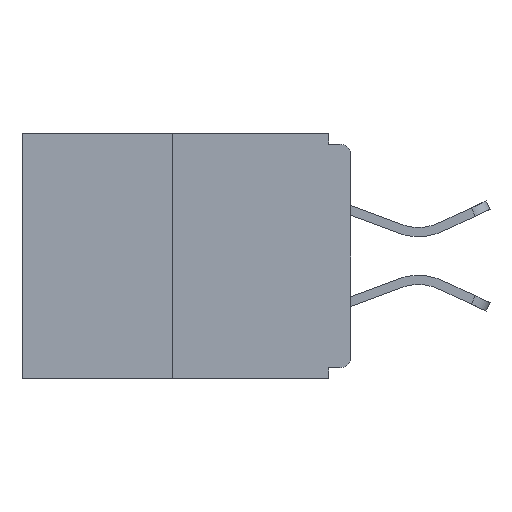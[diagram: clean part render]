
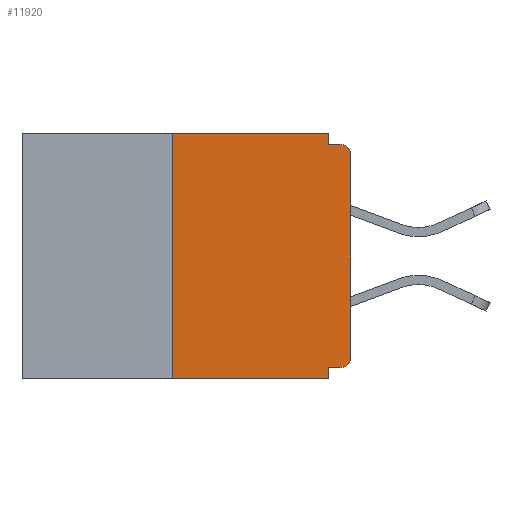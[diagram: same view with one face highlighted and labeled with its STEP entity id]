
A CAD part, left-side view. The second image highlights one B-rep face of the part: STEP entity #11920.
In plain terms, the highlighted planar face has unit normal (-1, 0, 0).
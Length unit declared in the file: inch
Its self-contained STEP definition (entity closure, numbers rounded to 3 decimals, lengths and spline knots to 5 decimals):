
#701 = CIRCLE ( 'NONE', #27333, 0.015 ) ;
#1292 = VERTEX_POINT ( 'NONE', #9075 ) ;
#2211 = CARTESIAN_POINT ( 'NONE',  ( 0., 0.25, 0. ) ) ;
#2224 = CARTESIAN_POINT ( 'NONE',  ( 0., 0.031, -0.015 ) ) ;
#3467 = VERTEX_POINT ( 'NONE', #19115 ) ;
#3936 = EDGE_CURVE ( 'NONE', #1292, #20335, #16505, .T. ) ;
#4167 = EDGE_CURVE ( 'NONE', #28776, #17093, #6380, .T. ) ;
#4776 = CARTESIAN_POINT ( 'NONE',  ( 0., 0.031, 0. ) ) ;
#5750 = CIRCLE ( 'NONE', #9636, 0.015 ) ;
#6220 = DIRECTION ( 'NONE',  ( 0., 0., 1. ) ) ;
#6380 = LINE ( 'NONE', #16462, #31080 ) ;
#6682 = CARTESIAN_POINT ( 'NONE',  ( 0., 0.031, 0. ) ) ;
#6690 = EDGE_CURVE ( 'NONE', #9240, #1292, #701, .T. ) ;
#6781 = VECTOR ( 'NONE', #25432, 39.37008 ) ;
#7291 = ORIENTED_EDGE ( 'NONE', *, *, #4167, .T. ) ;
#7718 = EDGE_CURVE ( 'NONE', #3467, #17093, #22141, .T. ) ;
#8162 = VECTOR ( 'NONE', #19704, 39.37008 ) ;
#8399 = LINE ( 'NONE', #25861, #15751 ) ;
#9075 = CARTESIAN_POINT ( 'NONE',  ( 0., 0., -0.313 ) ) ;
#9240 = VERTEX_POINT ( 'NONE', #25787 ) ;
#9314 = EDGE_CURVE ( 'NONE', #31200, #23020, #10562, .T. ) ;
#9426 = CARTESIAN_POINT ( 'NONE',  ( 0., 0.015, -0.313 ) ) ;
#9548 = CARTESIAN_POINT ( 'NONE',  ( 0., 0.031, -0.343 ) ) ;
#9636 = AXIS2_PLACEMENT_3D ( 'NONE', #28320, #13290, #18084 ) ;
#10562 = LINE ( 'NONE', #6682, #29783 ) ;
#11920 = ADVANCED_FACE ( 'NONE', ( #14346 ), #28567, .F. ) ;
#12516 = ORIENTED_EDGE ( 'NONE', *, *, #15513, .F. ) ;
#13290 = DIRECTION ( 'NONE',  ( -1., 0., 0. ) ) ;
#13300 = CARTESIAN_POINT ( 'NONE',  ( 0., 0.46, 0. ) ) ;
#13305 = VERTEX_POINT ( 'NONE', #31571 ) ;
#13986 = DIRECTION ( 'NONE',  ( 1., 0., 0. ) ) ;
#14346 = FACE_OUTER_BOUND ( 'NONE', #15248, .T. ) ;
#14464 = AXIS2_PLACEMENT_3D ( 'NONE', #26208, #13986, #16027 ) ;
#15248 = EDGE_LOOP ( 'NONE', ( #20607, #30064, #7291, #23464, #16384, #20181, #25159, #20839, #12516, #31578 ) ) ;
#15513 = EDGE_CURVE ( 'NONE', #23020, #13305, #8399, .T. ) ;
#15751 = VECTOR ( 'NONE', #30982, 39.37008 ) ;
#15843 = VERTEX_POINT ( 'NONE', #2211 ) ;
#16027 = DIRECTION ( 'NONE',  ( 0., 0., -1. ) ) ;
#16252 = EDGE_CURVE ( 'NONE', #15843, #31200, #31839, .T. ) ;
#16319 = DIRECTION ( 'NONE',  ( 0., 0., -1. ) ) ;
#16384 = ORIENTED_EDGE ( 'NONE', *, *, #29348, .F. ) ;
#16462 = CARTESIAN_POINT ( 'NONE',  ( 0., 0.46, -0.343 ) ) ;
#16505 = LINE ( 'NONE', #31599, #29852 ) ;
#17093 = VERTEX_POINT ( 'NONE', #9548 ) ;
#17262 = CARTESIAN_POINT ( 'NONE',  ( 0., 0.25, 0. ) ) ;
#18084 = DIRECTION ( 'NONE',  ( 0., 0., -1. ) ) ;
#18687 = DIRECTION ( 'NONE',  ( 0., 0., -1. ) ) ;
#18782 = DIRECTION ( 'NONE',  ( 0., 1., 0. ) ) ;
#19115 = CARTESIAN_POINT ( 'NONE',  ( 0., 0.031, -0.328 ) ) ;
#19704 = DIRECTION ( 'NONE',  ( 0., 0., 1. ) ) ;
#20181 = ORIENTED_EDGE ( 'NONE', *, *, #6690, .T. ) ;
#20218 = EDGE_CURVE ( 'NONE', #20335, #13305, #5750, .T. ) ;
#20232 = LINE ( 'NONE', #17262, #8162 ) ;
#20335 = VERTEX_POINT ( 'NONE', #24767 ) ;
#20580 = VECTOR ( 'NONE', #16319, 39.37008 ) ;
#20607 = ORIENTED_EDGE ( 'NONE', *, *, #16252, .F. ) ;
#20839 = ORIENTED_EDGE ( 'NONE', *, *, #20218, .T. ) ;
#21516 = DIRECTION ( 'NONE',  ( 0., -1., 0. ) ) ;
#22141 = LINE ( 'NONE', #30966, #20580 ) ;
#23020 = VERTEX_POINT ( 'NONE', #2224 ) ;
#23464 = ORIENTED_EDGE ( 'NONE', *, *, #7718, .F. ) ;
#23481 = CARTESIAN_POINT ( 'NONE',  ( 0., 0., -0.328 ) ) ;
#24767 = CARTESIAN_POINT ( 'NONE',  ( 0., 0., -0.03 ) ) ;
#25159 = ORIENTED_EDGE ( 'NONE', *, *, #3936, .T. ) ;
#25432 = DIRECTION ( 'NONE',  ( 0., -1., 0. ) ) ;
#25787 = CARTESIAN_POINT ( 'NONE',  ( 0., 0.015, -0.328 ) ) ;
#25789 = VECTOR ( 'NONE', #18782, 39.37008 ) ;
#25861 = CARTESIAN_POINT ( 'NONE',  ( 0., 0., -0.015 ) ) ;
#26208 = CARTESIAN_POINT ( 'NONE',  ( 0., 0.46, 0. ) ) ;
#27029 = CARTESIAN_POINT ( 'NONE',  ( 0., 0.25, -0.343 ) ) ;
#27333 = AXIS2_PLACEMENT_3D ( 'NONE', #9426, #27467, #31881 ) ;
#27467 = DIRECTION ( 'NONE',  ( -1., 0., 0. ) ) ;
#28320 = CARTESIAN_POINT ( 'NONE',  ( 0., 0.015, -0.03 ) ) ;
#28567 = PLANE ( 'NONE',  #14464 ) ;
#28776 = VERTEX_POINT ( 'NONE', #27029 ) ;
#29348 = EDGE_CURVE ( 'NONE', #9240, #3467, #30166, .T. ) ;
#29783 = VECTOR ( 'NONE', #18687, 39.37008 ) ;
#29852 = VECTOR ( 'NONE', #6220, 39.37008 ) ;
#30064 = ORIENTED_EDGE ( 'NONE', *, *, #31263, .F. ) ;
#30166 = LINE ( 'NONE', #23481, #25789 ) ;
#30966 = CARTESIAN_POINT ( 'NONE',  ( 0., 0.031, -0.343 ) ) ;
#30982 = DIRECTION ( 'NONE',  ( 0., -1., 0. ) ) ;
#31080 = VECTOR ( 'NONE', #21516, 39.37008 ) ;
#31200 = VERTEX_POINT ( 'NONE', #4776 ) ;
#31263 = EDGE_CURVE ( 'NONE', #28776, #15843, #20232, .T. ) ;
#31571 = CARTESIAN_POINT ( 'NONE',  ( 0., 0.015, -0.015 ) ) ;
#31578 = ORIENTED_EDGE ( 'NONE', *, *, #9314, .F. ) ;
#31599 = CARTESIAN_POINT ( 'NONE',  ( 0., 0., 0. ) ) ;
#31839 = LINE ( 'NONE', #13300, #6781 ) ;
#31881 = DIRECTION ( 'NONE',  ( 0., 0., -1. ) ) ;
